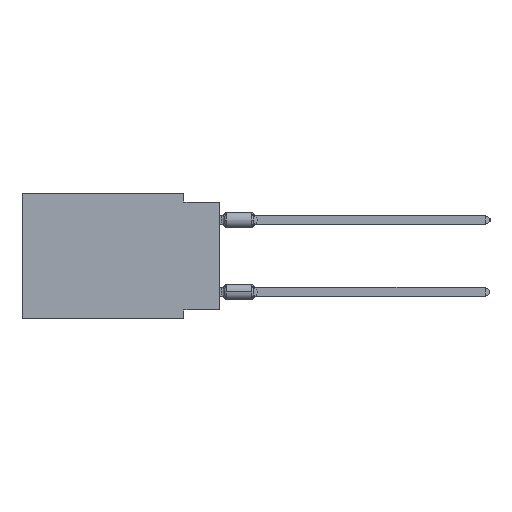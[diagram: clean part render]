
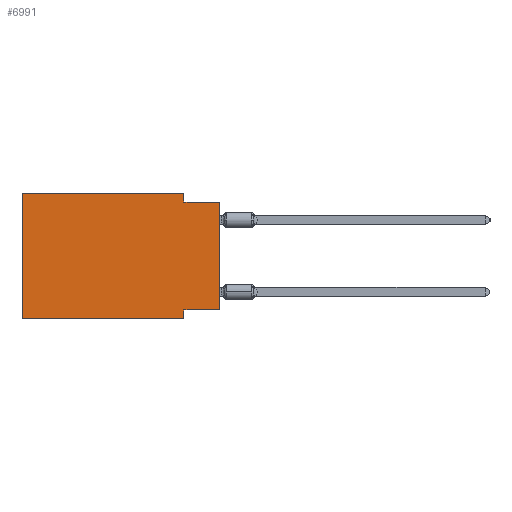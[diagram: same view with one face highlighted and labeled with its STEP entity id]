
A CAD part, left-side view. The second image highlights one B-rep face of the part: STEP entity #6991.
In plain terms, the highlighted planar face has unit normal (-1, 0, 0).
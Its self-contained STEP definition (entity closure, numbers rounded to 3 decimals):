
#381 = VERTEX_POINT ( 'NONE', #17193 ) ;
#605 = ORIENTED_EDGE ( 'NONE', *, *, #21996, .F. ) ;
#1301 = ORIENTED_EDGE ( 'NONE', *, *, #7543, .T. ) ;
#1384 = VECTOR ( 'NONE', #17454, 1000. ) ;
#1883 = ORIENTED_EDGE ( 'NONE', *, *, #10824, .T. ) ;
#2129 = EDGE_CURVE ( 'NONE', #22984, #8888, #2776, .T. ) ;
#2672 = CARTESIAN_POINT ( 'NONE',  ( 0., 13.97, -8.89 ) ) ;
#2776 = LINE ( 'NONE', #5271, #24041 ) ;
#2815 = EDGE_LOOP ( 'NONE', ( #1301, #18608, #605, #25152, #23594, #1883, #17852, #25488 ) ) ;
#3203 = LINE ( 'NONE', #16703, #21992 ) ;
#3545 = CARTESIAN_POINT ( 'NONE',  ( 0., 0., -0.635 ) ) ;
#3934 = CARTESIAN_POINT ( 'NONE',  ( 0., 2.54, -8.89 ) ) ;
#4826 = EDGE_CURVE ( 'NONE', #8888, #10663, #3203, .T. ) ;
#5076 = CARTESIAN_POINT ( 'NONE',  ( 0., 0., -0.635 ) ) ;
#5271 = CARTESIAN_POINT ( 'NONE',  ( 0., 0., -8.255 ) ) ;
#6167 = AXIS2_PLACEMENT_3D ( 'NONE', #11799, #13600, #13464 ) ;
#6343 = LINE ( 'NONE', #12960, #8967 ) ;
#6357 = VERTEX_POINT ( 'NONE', #21571 ) ;
#6554 = LINE ( 'NONE', #2672, #1384 ) ;
#6783 = CARTESIAN_POINT ( 'NONE',  ( 0., 2.54, -8.255 ) ) ;
#6991 = ADVANCED_FACE ( 'NONE', ( #7653 ), #24544, .F. ) ;
#7543 = EDGE_CURVE ( 'NONE', #22984, #19982, #16186, .T. ) ;
#7653 = FACE_OUTER_BOUND ( 'NONE', #2815, .T. ) ;
#8385 = EDGE_CURVE ( 'NONE', #6357, #19982, #22360, .T. ) ;
#8888 = VERTEX_POINT ( 'NONE', #6783 ) ;
#8963 = VECTOR ( 'NONE', #15996, 1000. ) ;
#8967 = VECTOR ( 'NONE', #12696, 1000. ) ;
#10022 = CARTESIAN_POINT ( 'NONE',  ( 0., 0., -8.255 ) ) ;
#10663 = VERTEX_POINT ( 'NONE', #3934 ) ;
#10824 = EDGE_CURVE ( 'NONE', #21101, #10663, #6554, .T. ) ;
#11303 = LINE ( 'NONE', #19884, #8963 ) ;
#11698 = DIRECTION ( 'NONE',  ( 0., -1., 0. ) ) ;
#11799 = CARTESIAN_POINT ( 'NONE',  ( 0., 13.97, 0. ) ) ;
#11855 = CARTESIAN_POINT ( 'NONE',  ( 0., 13.97, 0. ) ) ;
#12696 = DIRECTION ( 'NONE',  ( 0., 0., 1. ) ) ;
#12960 = CARTESIAN_POINT ( 'NONE',  ( 0., 13.97, 0. ) ) ;
#12964 = EDGE_CURVE ( 'NONE', #25173, #381, #11303, .T. ) ;
#13464 = DIRECTION ( 'NONE',  ( 0., 0., -1. ) ) ;
#13600 = DIRECTION ( 'NONE',  ( 1., 0., 0. ) ) ;
#15030 = CARTESIAN_POINT ( 'NONE',  ( 0., 13.97, -8.89 ) ) ;
#15996 = DIRECTION ( 'NONE',  ( 0., -1., 0. ) ) ;
#16186 = LINE ( 'NONE', #22978, #26009 ) ;
#16703 = CARTESIAN_POINT ( 'NONE',  ( 0., 2.54, -8.89 ) ) ;
#17193 = CARTESIAN_POINT ( 'NONE',  ( 0., 2.54, 0. ) ) ;
#17454 = DIRECTION ( 'NONE',  ( 0., -1., 0. ) ) ;
#17852 = ORIENTED_EDGE ( 'NONE', *, *, #4826, .F. ) ;
#18608 = ORIENTED_EDGE ( 'NONE', *, *, #8385, .F. ) ;
#18990 = LINE ( 'NONE', #23278, #26027 ) ;
#19884 = CARTESIAN_POINT ( 'NONE',  ( 0., 13.97, 0. ) ) ;
#19982 = VERTEX_POINT ( 'NONE', #5076 ) ;
#20272 = VECTOR ( 'NONE', #11698, 1000. ) ;
#21101 = VERTEX_POINT ( 'NONE', #15030 ) ;
#21571 = CARTESIAN_POINT ( 'NONE',  ( 0., 2.54, -0.635 ) ) ;
#21992 = VECTOR ( 'NONE', #24506, 1000. ) ;
#21996 = EDGE_CURVE ( 'NONE', #381, #6357, #18990, .T. ) ;
#22360 = LINE ( 'NONE', #3545, #20272 ) ;
#22978 = CARTESIAN_POINT ( 'NONE',  ( 0., 0., 0. ) ) ;
#22984 = VERTEX_POINT ( 'NONE', #10022 ) ;
#23278 = CARTESIAN_POINT ( 'NONE',  ( 0., 2.54, 0. ) ) ;
#23422 = DIRECTION ( 'NONE',  ( 0., 0., -1. ) ) ;
#23594 = ORIENTED_EDGE ( 'NONE', *, *, #27175, .F. ) ;
#24041 = VECTOR ( 'NONE', #26300, 1000. ) ;
#24506 = DIRECTION ( 'NONE',  ( 0., 0., -1. ) ) ;
#24510 = DIRECTION ( 'NONE',  ( 0., 0., 1. ) ) ;
#24544 = PLANE ( 'NONE',  #6167 ) ;
#25152 = ORIENTED_EDGE ( 'NONE', *, *, #12964, .F. ) ;
#25173 = VERTEX_POINT ( 'NONE', #11855 ) ;
#25488 = ORIENTED_EDGE ( 'NONE', *, *, #2129, .F. ) ;
#26009 = VECTOR ( 'NONE', #24510, 1000. ) ;
#26027 = VECTOR ( 'NONE', #23422, 1000. ) ;
#26300 = DIRECTION ( 'NONE',  ( 0., 1., 0. ) ) ;
#27175 = EDGE_CURVE ( 'NONE', #21101, #25173, #6343, .T. ) ;
